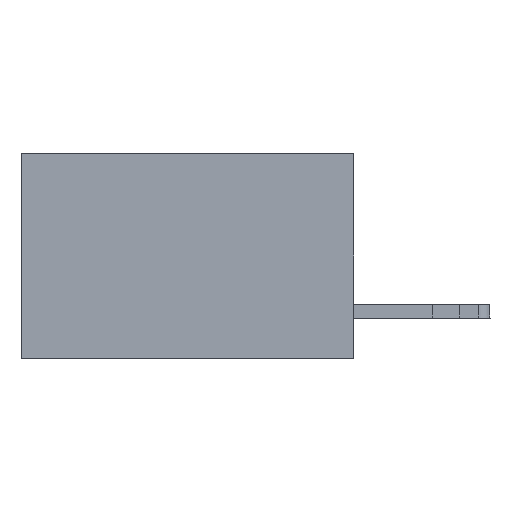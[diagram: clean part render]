
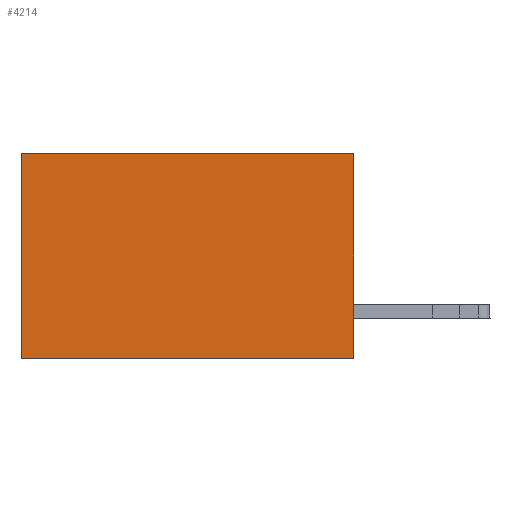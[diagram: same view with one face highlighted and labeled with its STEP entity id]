
A CAD part, left-side view. The second image highlights one B-rep face of the part: STEP entity #4214.
In plain terms, the highlighted planar face has unit normal (-1, 0, 0).
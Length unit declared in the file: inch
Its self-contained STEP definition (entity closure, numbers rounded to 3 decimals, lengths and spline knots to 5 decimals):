
#1514 = EDGE_LOOP ( 'NONE', ( #17500, #18812, #3513, #3207 ) ) ;
#2285 = CARTESIAN_POINT ( 'NONE',  ( 0.2875, 0., 0. ) ) ;
#3207 = ORIENTED_EDGE ( 'NONE', *, *, #5968, .T. ) ;
#3513 = ORIENTED_EDGE ( 'NONE', *, *, #13116, .F. ) ;
#4214 = ADVANCED_FACE ( 'NONE', ( #21126 ), #6317, .F. ) ;
#4744 = VERTEX_POINT ( 'NONE', #6578 ) ;
#4905 = CARTESIAN_POINT ( 'NONE',  ( 0.2875, 0., -0.37 ) ) ;
#5210 = LINE ( 'NONE', #2285, #19281 ) ;
#5968 = EDGE_CURVE ( 'NONE', #6328, #21317, #13999, .T. ) ;
#6317 = PLANE ( 'NONE',  #19469 ) ;
#6328 = VERTEX_POINT ( 'NONE', #18767 ) ;
#6578 = CARTESIAN_POINT ( 'NONE',  ( 0.2875, 0.6, -0.37 ) ) ;
#6981 = LINE ( 'NONE', #7153, #19215 ) ;
#7153 = CARTESIAN_POINT ( 'NONE',  ( 0.2875, 0.6, 0. ) ) ;
#7803 = VECTOR ( 'NONE', #18447, 39.37008 ) ;
#7910 = CARTESIAN_POINT ( 'NONE',  ( 0.2875, 0., -0.37 ) ) ;
#8109 = DIRECTION ( 'NONE',  ( 1., 0., 0. ) ) ;
#8942 = DIRECTION ( 'NONE',  ( 0., 0., -1. ) ) ;
#9207 = CARTESIAN_POINT ( 'NONE',  ( 0.2875, 0., 0. ) ) ;
#11432 = DIRECTION ( 'NONE',  ( 0., 0., -1. ) ) ;
#12361 = DIRECTION ( 'NONE',  ( 0., 0., -1. ) ) ;
#13116 = EDGE_CURVE ( 'NONE', #6328, #13256, #5210, .T. ) ;
#13256 = VERTEX_POINT ( 'NONE', #4905 ) ;
#13999 = LINE ( 'NONE', #19570, #19850 ) ;
#14660 = EDGE_CURVE ( 'NONE', #13256, #4744, #17895, .T. ) ;
#14951 = EDGE_CURVE ( 'NONE', #21317, #4744, #6981, .T. ) ;
#16483 = CARTESIAN_POINT ( 'NONE',  ( 0.2875, 0.6, 0. ) ) ;
#17500 = ORIENTED_EDGE ( 'NONE', *, *, #14951, .T. ) ;
#17731 = DIRECTION ( 'NONE',  ( 0., 1., 0. ) ) ;
#17895 = LINE ( 'NONE', #7910, #7803 ) ;
#18447 = DIRECTION ( 'NONE',  ( 0., 1., 0. ) ) ;
#18767 = CARTESIAN_POINT ( 'NONE',  ( 0.2875, 0., 0. ) ) ;
#18812 = ORIENTED_EDGE ( 'NONE', *, *, #14660, .F. ) ;
#19215 = VECTOR ( 'NONE', #12361, 39.37008 ) ;
#19281 = VECTOR ( 'NONE', #8942, 39.37008 ) ;
#19469 = AXIS2_PLACEMENT_3D ( 'NONE', #9207, #8109, #11432 ) ;
#19570 = CARTESIAN_POINT ( 'NONE',  ( 0.2875, 0., 0. ) ) ;
#19850 = VECTOR ( 'NONE', #17731, 39.37008 ) ;
#21126 = FACE_OUTER_BOUND ( 'NONE', #1514, .T. ) ;
#21317 = VERTEX_POINT ( 'NONE', #16483 ) ;
